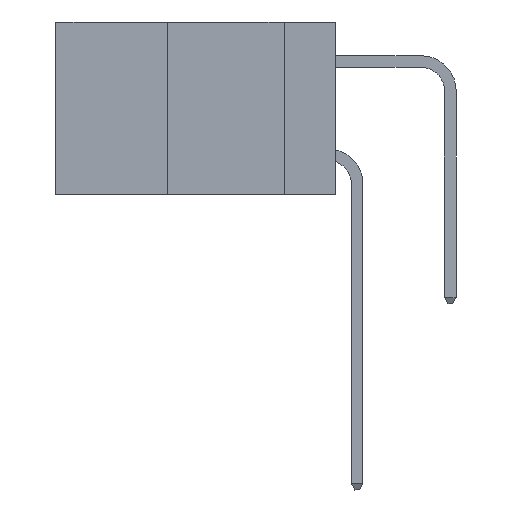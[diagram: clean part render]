
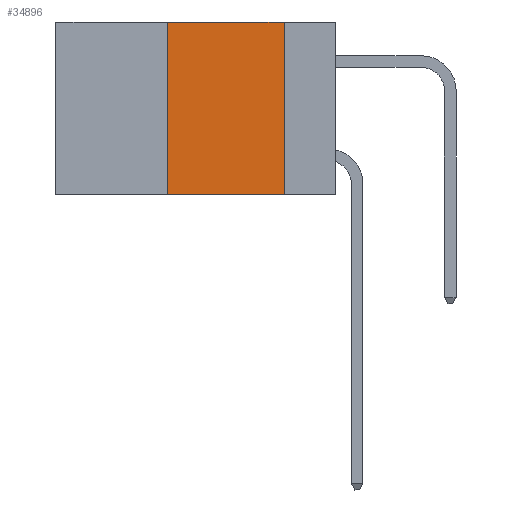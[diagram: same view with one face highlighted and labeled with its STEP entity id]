
A CAD part, left-side view. The second image highlights one B-rep face of the part: STEP entity #34896.
In plain terms, the highlighted planar face has unit normal (-1, 0, 0).
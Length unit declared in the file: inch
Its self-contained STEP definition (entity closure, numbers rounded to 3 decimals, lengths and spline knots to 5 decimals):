
#1751 = CARTESIAN_POINT ( 'NONE',  ( 0., 0.11, 0. ) ) ;
#6206 = EDGE_CURVE ( 'NONE', #26836, #32407, #41650, .T. ) ;
#6531 = LINE ( 'NONE', #22345, #17972 ) ;
#6840 = CARTESIAN_POINT ( 'NONE',  ( 0., 0.11, 0. ) ) ;
#8427 = FACE_OUTER_BOUND ( 'NONE', #39772, .T. ) ;
#8728 = ORIENTED_EDGE ( 'NONE', *, *, #42317, .F. ) ;
#8886 = VECTOR ( 'NONE', #38890, 39.37008 ) ;
#9195 = VECTOR ( 'NONE', #14520, 39.37008 ) ;
#9961 = ORIENTED_EDGE ( 'NONE', *, *, #31075, .F. ) ;
#10116 = ORIENTED_EDGE ( 'NONE', *, *, #18699, .T. ) ;
#12372 = CARTESIAN_POINT ( 'NONE',  ( 0., 0.6, 0. ) ) ;
#14487 = ORIENTED_EDGE ( 'NONE', *, *, #6206, .F. ) ;
#14520 = DIRECTION ( 'NONE',  ( 0., -1., 0. ) ) ;
#16704 = VECTOR ( 'NONE', #34820, 39.37008 ) ;
#17951 = PLANE ( 'NONE',  #36486 ) ;
#17972 = VECTOR ( 'NONE', #33257, 39.37008 ) ;
#18699 = EDGE_CURVE ( 'NONE', #39660, #33627, #29220, .T. ) ;
#20747 = DIRECTION ( 'NONE',  ( 1., 0., 0. ) ) ;
#22345 = CARTESIAN_POINT ( 'NONE',  ( 0., 0.36, 0. ) ) ;
#25612 = LINE ( 'NONE', #1751, #16704 ) ;
#26661 = CARTESIAN_POINT ( 'NONE',  ( 0., 0.36, -0.37 ) ) ;
#26836 = VERTEX_POINT ( 'NONE', #42207 ) ;
#27861 = CARTESIAN_POINT ( 'NONE',  ( 0., 0.6, 0. ) ) ;
#29220 = LINE ( 'NONE', #39168, #8886 ) ;
#31075 = EDGE_CURVE ( 'NONE', #39660, #26836, #6531, .T. ) ;
#31089 = DIRECTION ( 'NONE',  ( 0., 0., -1. ) ) ;
#32407 = VERTEX_POINT ( 'NONE', #6840 ) ;
#33257 = DIRECTION ( 'NONE',  ( 0., 0., 1. ) ) ;
#33627 = VERTEX_POINT ( 'NONE', #41461 ) ;
#34820 = DIRECTION ( 'NONE',  ( 0., 0., -1. ) ) ;
#34896 = ADVANCED_FACE ( 'NONE', ( #8427 ), #17951, .F. ) ;
#36486 = AXIS2_PLACEMENT_3D ( 'NONE', #27861, #20747, #31089 ) ;
#38890 = DIRECTION ( 'NONE',  ( 0., -1., 0. ) ) ;
#39168 = CARTESIAN_POINT ( 'NONE',  ( 0., 0.6, -0.37 ) ) ;
#39660 = VERTEX_POINT ( 'NONE', #26661 ) ;
#39772 = EDGE_LOOP ( 'NONE', ( #8728, #14487, #9961, #10116 ) ) ;
#41461 = CARTESIAN_POINT ( 'NONE',  ( 0., 0.11, -0.37 ) ) ;
#41650 = LINE ( 'NONE', #12372, #9195 ) ;
#42207 = CARTESIAN_POINT ( 'NONE',  ( 0., 0.36, 0. ) ) ;
#42317 = EDGE_CURVE ( 'NONE', #32407, #33627, #25612, .T. ) ;
